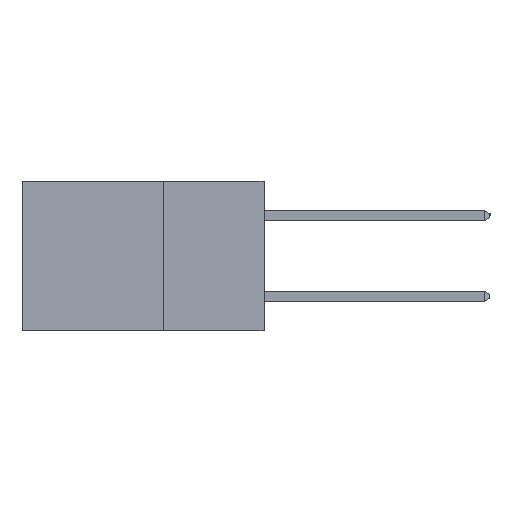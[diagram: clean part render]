
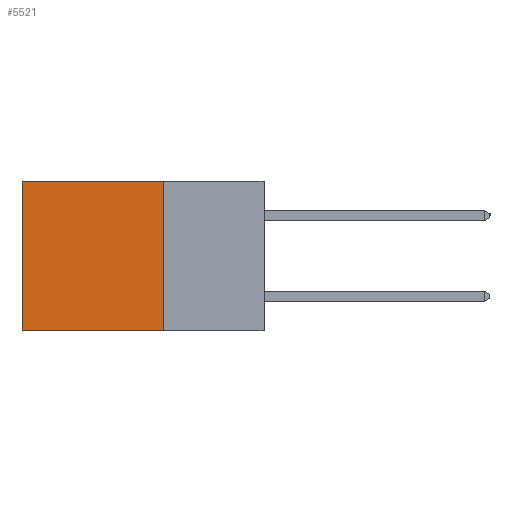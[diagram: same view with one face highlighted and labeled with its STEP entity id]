
A CAD part, left-side view. The second image highlights one B-rep face of the part: STEP entity #5521.
In plain terms, the highlighted planar face has unit normal (-1, 0, 0).
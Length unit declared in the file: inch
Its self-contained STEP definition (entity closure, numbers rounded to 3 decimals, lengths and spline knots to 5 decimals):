
#1162 = VERTEX_POINT ( 'NONE', #1698 ) ;
#1698 = CARTESIAN_POINT ( 'NONE',  ( 0.2615, 0.6, -0.37 ) ) ;
#1906 = CARTESIAN_POINT ( 'NONE',  ( 0.2615, 0.25, 0. ) ) ;
#3631 = VECTOR ( 'NONE', #13982, 39.37008 ) ;
#3735 = CARTESIAN_POINT ( 'NONE',  ( 0.2615, 0.25, -0.37 ) ) ;
#3778 = VECTOR ( 'NONE', #10610, 39.37008 ) ;
#3957 = ORIENTED_EDGE ( 'NONE', *, *, #9054, .T. ) ;
#4272 = PLANE ( 'NONE',  #13849 ) ;
#4488 = LINE ( 'NONE', #9532, #3778 ) ;
#5521 = ADVANCED_FACE ( 'NONE', ( #14499 ), #4272, .F. ) ;
#5668 = CARTESIAN_POINT ( 'NONE',  ( 0.2615, 0.6, 0. ) ) ;
#5682 = DIRECTION ( 'NONE',  ( 0., 0., -1. ) ) ;
#6277 = EDGE_LOOP ( 'NONE', ( #11817, #9414, #8234, #3957 ) ) ;
#7003 = DIRECTION ( 'NONE',  ( 1., 0., 0. ) ) ;
#7472 = LINE ( 'NONE', #7553, #9444 ) ;
#7553 = CARTESIAN_POINT ( 'NONE',  ( 0.2615, 0.25, -0.37 ) ) ;
#8234 = ORIENTED_EDGE ( 'NONE', *, *, #16144, .F. ) ;
#9054 = EDGE_CURVE ( 'NONE', #9970, #10588, #4488, .T. ) ;
#9308 = CARTESIAN_POINT ( 'NONE',  ( 0.2615, 0.25, -0.37 ) ) ;
#9406 = VERTEX_POINT ( 'NONE', #3735 ) ;
#9414 = ORIENTED_EDGE ( 'NONE', *, *, #16041, .F. ) ;
#9444 = VECTOR ( 'NONE', #16202, 39.37008 ) ;
#9532 = CARTESIAN_POINT ( 'NONE',  ( 0.2615, 0.25, 0. ) ) ;
#9970 = VERTEX_POINT ( 'NONE', #1906 ) ;
#10287 = CARTESIAN_POINT ( 'NONE',  ( 0.2615, 0.25, -0.37 ) ) ;
#10446 = VECTOR ( 'NONE', #14828, 39.37008 ) ;
#10588 = VERTEX_POINT ( 'NONE', #5668 ) ;
#10610 = DIRECTION ( 'NONE',  ( 0., 1., 0. ) ) ;
#11062 = CARTESIAN_POINT ( 'NONE',  ( 0.2615, 0.6, -0.37 ) ) ;
#11214 = LINE ( 'NONE', #11062, #10446 ) ;
#11750 = LINE ( 'NONE', #10287, #3631 ) ;
#11817 = ORIENTED_EDGE ( 'NONE', *, *, #12330, .T. ) ;
#12330 = EDGE_CURVE ( 'NONE', #10588, #1162, #11214, .T. ) ;
#13849 = AXIS2_PLACEMENT_3D ( 'NONE', #9308, #7003, #5682 ) ;
#13982 = DIRECTION ( 'NONE',  ( 0., 0., -1. ) ) ;
#14499 = FACE_OUTER_BOUND ( 'NONE', #6277, .T. ) ;
#14828 = DIRECTION ( 'NONE',  ( 0., 0., -1. ) ) ;
#16041 = EDGE_CURVE ( 'NONE', #9406, #1162, #7472, .T. ) ;
#16144 = EDGE_CURVE ( 'NONE', #9970, #9406, #11750, .T. ) ;
#16202 = DIRECTION ( 'NONE',  ( 0., 1., 0. ) ) ;
